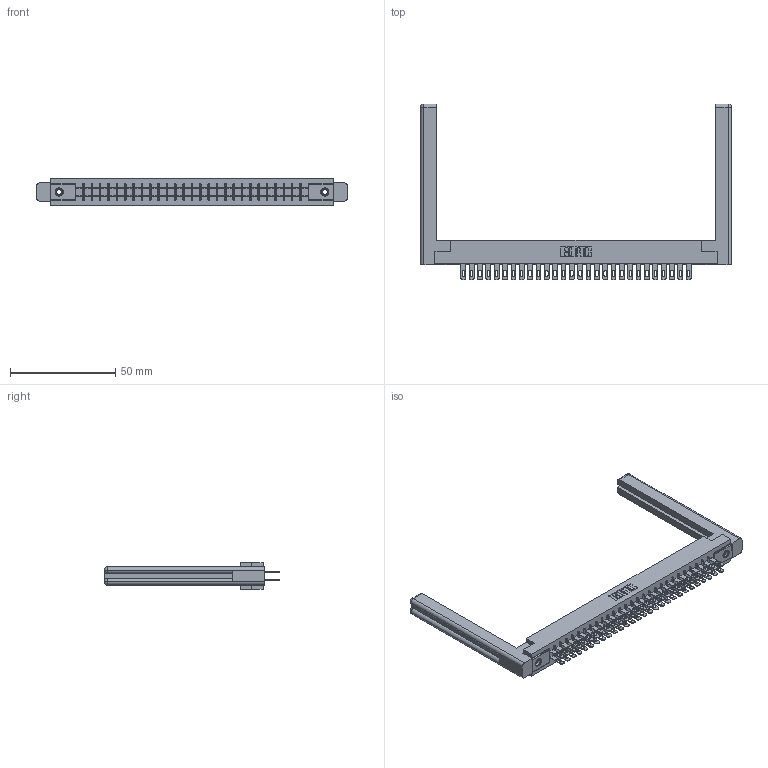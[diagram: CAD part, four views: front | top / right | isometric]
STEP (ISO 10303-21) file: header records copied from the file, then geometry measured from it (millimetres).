
FILE_DESCRIPTION (( 'STEP AP203' ), '1' );
FILE_NAME ('305-056-500-258.STEP', '2019-09-09T23:27:40', ( '' ), ( '' ), 'SwSTEP 2.0', 'SolidWorks 2016', '' );
FILE_SCHEMA (( 'CONFIG_CONTROL_DESIGN' ));
Length unit declared in the file: inch
Products named in the file (5): 345-250-001_345-250-001-102; 305-290-001_500; 305 Part_.156 Dia; 305-056-500-258; 307-220-058
Assembly tree (61 placements, depth 2):
  305-056-500-258
    305 Part_.156 Dia
    305-290-001_500  x56
    345-250-001_345-250-001-102  x2
    307-220-058  x2
Bounding box: 147.57 x 83.49 x 12.7 mm (x, y, z)
Volume: 22637.4 mm3; surface area: 25335.5 mm2
Topology: 61 solids, 61 shells, 3058 faces, 8706 edges, 5640 vertices
Faces by surface type: plane 1720, cylinder 1202, sphere 112, cone 12, torus 12
Entity records: 34676 total; most frequent: CARTESIAN_POINT 5753, ORIENTED_EDGE 5650, DIRECTION 5541, EDGE_CURVE 2825, VECTOR 2257, LINE 2257, VERTEX_POINT 1800, AXIS2_PLACEMENT_3D 1642
